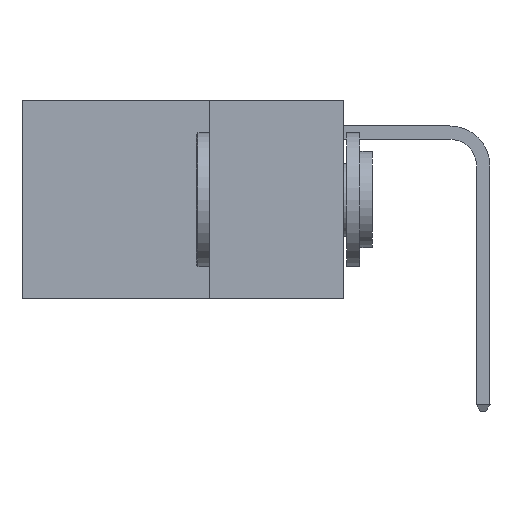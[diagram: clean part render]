
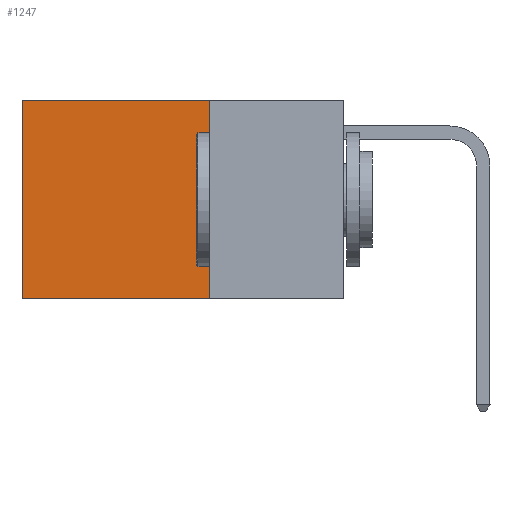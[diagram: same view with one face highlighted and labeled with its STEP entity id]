
A CAD part, left-side view. The second image highlights one B-rep face of the part: STEP entity #1247.
In plain terms, the highlighted planar face has unit normal (-1, 0, 0).
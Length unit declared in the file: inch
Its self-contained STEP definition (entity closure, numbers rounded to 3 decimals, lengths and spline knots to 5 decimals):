
#412 = DIRECTION ( 'NONE',  ( 0., 0., -1. ) ) ;
#1215 = VERTEX_POINT ( 'NONE', #7218 ) ;
#1239 = CARTESIAN_POINT ( 'NONE',  ( 0.2625, 0.25, 0. ) ) ;
#1247 = ADVANCED_FACE ( 'NONE', ( #3691 ), #6861, .F. ) ;
#1719 = DIRECTION ( 'NONE',  ( 0., 0., -1. ) ) ;
#2139 = CARTESIAN_POINT ( 'NONE',  ( 0.2625, 0.6, 0. ) ) ;
#2957 = CARTESIAN_POINT ( 'NONE',  ( 0.2625, 0.25, 0. ) ) ;
#3073 = ORIENTED_EDGE ( 'NONE', *, *, #3635, .T. ) ;
#3437 = LINE ( 'NONE', #9711, #3832 ) ;
#3635 = EDGE_CURVE ( 'NONE', #14885, #7442, #7186, .T. ) ;
#3691 = FACE_OUTER_BOUND ( 'NONE', #15251, .T. ) ;
#3832 = VECTOR ( 'NONE', #15982, 39.37008 ) ;
#5133 = CARTESIAN_POINT ( 'NONE',  ( 0.2625, 0.6, 0. ) ) ;
#6357 = DIRECTION ( 'NONE',  ( 1., 0., 0. ) ) ;
#6462 = CARTESIAN_POINT ( 'NONE',  ( 0.2625, 0.25, 0. ) ) ;
#6861 = PLANE ( 'NONE',  #10700 ) ;
#7169 = VECTOR ( 'NONE', #1719, 39.37008 ) ;
#7186 = LINE ( 'NONE', #2139, #7169 ) ;
#7218 = CARTESIAN_POINT ( 'NONE',  ( 0.2625, 0.25, -0.37 ) ) ;
#7442 = VERTEX_POINT ( 'NONE', #12357 ) ;
#7801 = EDGE_CURVE ( 'NONE', #13762, #1215, #12224, .T. ) ;
#8176 = DIRECTION ( 'NONE',  ( 0., 0., -1. ) ) ;
#8241 = CARTESIAN_POINT ( 'NONE',  ( 0.2625, 0.25, 0. ) ) ;
#8472 = VECTOR ( 'NONE', #15619, 39.37008 ) ;
#8858 = LINE ( 'NONE', #2957, #8472 ) ;
#8991 = ORIENTED_EDGE ( 'NONE', *, *, #14565, .T. ) ;
#9711 = CARTESIAN_POINT ( 'NONE',  ( 0.2625, 0.25, -0.37 ) ) ;
#10700 = AXIS2_PLACEMENT_3D ( 'NONE', #6462, #6357, #412 ) ;
#10876 = ORIENTED_EDGE ( 'NONE', *, *, #13177, .F. ) ;
#12108 = VECTOR ( 'NONE', #8176, 39.37008 ) ;
#12224 = LINE ( 'NONE', #8241, #12108 ) ;
#12357 = CARTESIAN_POINT ( 'NONE',  ( 0.2625, 0.6, -0.37 ) ) ;
#13177 = EDGE_CURVE ( 'NONE', #1215, #7442, #3437, .T. ) ;
#13762 = VERTEX_POINT ( 'NONE', #1239 ) ;
#14565 = EDGE_CURVE ( 'NONE', #13762, #14885, #8858, .T. ) ;
#14885 = VERTEX_POINT ( 'NONE', #5133 ) ;
#15251 = EDGE_LOOP ( 'NONE', ( #3073, #10876, #16569, #8991 ) ) ;
#15619 = DIRECTION ( 'NONE',  ( 0., 1., 0. ) ) ;
#15982 = DIRECTION ( 'NONE',  ( 0., 1., 0. ) ) ;
#16569 = ORIENTED_EDGE ( 'NONE', *, *, #7801, .F. ) ;
